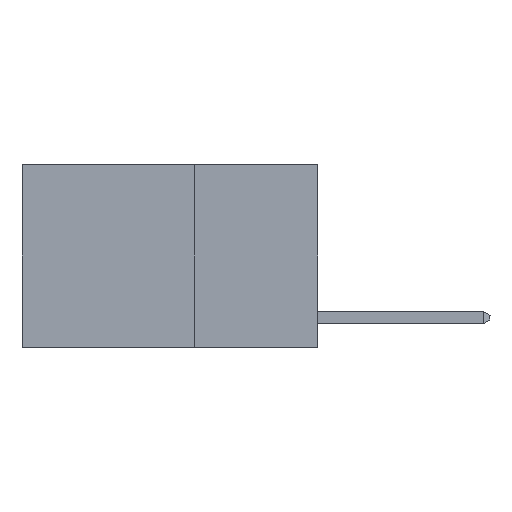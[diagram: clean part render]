
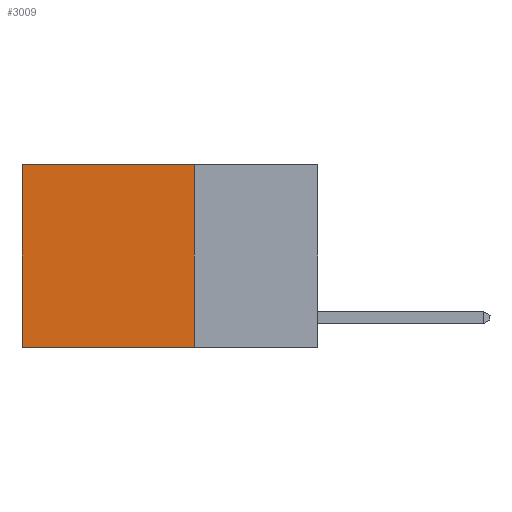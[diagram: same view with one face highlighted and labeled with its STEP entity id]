
A CAD part, left-side view. The second image highlights one B-rep face of the part: STEP entity #3009.
In plain terms, the highlighted planar face has unit normal (-1, 0, 0).
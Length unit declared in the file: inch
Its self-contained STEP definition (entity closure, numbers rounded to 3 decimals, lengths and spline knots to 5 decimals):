
#462 = LINE ( 'NONE', #7284, #9658 ) ;
#715 = VERTEX_POINT ( 'NONE', #5923 ) ;
#879 = AXIS2_PLACEMENT_3D ( 'NONE', #6379, #951, #7231 ) ;
#911 = EDGE_CURVE ( 'NONE', #4923, #715, #462, .T. ) ;
#945 = ORIENTED_EDGE ( 'NONE', *, *, #1492, .T. ) ;
#951 = DIRECTION ( 'NONE',  ( 1., 0., 0. ) ) ;
#1156 = LINE ( 'NONE', #4489, #3447 ) ;
#1469 = CARTESIAN_POINT ( 'NONE',  ( 0.2625, 0.6, 0. ) ) ;
#1492 = EDGE_CURVE ( 'NONE', #6433, #715, #4643, .T. ) ;
#1773 = EDGE_CURVE ( 'NONE', #6841, #4923, #7531, .T. ) ;
#1818 = VECTOR ( 'NONE', #6863, 39.37008 ) ;
#1923 = ORIENTED_EDGE ( 'NONE', *, *, #5623, .T. ) ;
#2501 = CARTESIAN_POINT ( 'NONE',  ( 0.2625, 0.25, 0. ) ) ;
#2544 = DIRECTION ( 'NONE',  ( 0., 0., -1. ) ) ;
#2850 = FACE_OUTER_BOUND ( 'NONE', #7343, .T. ) ;
#2915 = VECTOR ( 'NONE', #2544, 39.37008 ) ;
#3009 = ADVANCED_FACE ( 'NONE', ( #2850 ), #10342, .F. ) ;
#3053 = ORIENTED_EDGE ( 'NONE', *, *, #1773, .F. ) ;
#3447 = VECTOR ( 'NONE', #10206, 39.37008 ) ;
#4489 = CARTESIAN_POINT ( 'NONE',  ( 0.2625, 0.25, 0. ) ) ;
#4643 = LINE ( 'NONE', #7136, #1818 ) ;
#4923 = VERTEX_POINT ( 'NONE', #8606 ) ;
#5623 = EDGE_CURVE ( 'NONE', #6841, #6433, #1156, .T. ) ;
#5923 = CARTESIAN_POINT ( 'NONE',  ( 0.2625, 0.6, -0.37 ) ) ;
#6379 = CARTESIAN_POINT ( 'NONE',  ( 0.2625, 0.25, 0. ) ) ;
#6428 = DIRECTION ( 'NONE',  ( 0., 1., 0. ) ) ;
#6433 = VERTEX_POINT ( 'NONE', #1469 ) ;
#6841 = VERTEX_POINT ( 'NONE', #8933 ) ;
#6863 = DIRECTION ( 'NONE',  ( 0., 0., -1. ) ) ;
#7136 = CARTESIAN_POINT ( 'NONE',  ( 0.2625, 0.6, 0. ) ) ;
#7231 = DIRECTION ( 'NONE',  ( 0., 0., -1. ) ) ;
#7284 = CARTESIAN_POINT ( 'NONE',  ( 0.2625, 0.25, -0.37 ) ) ;
#7343 = EDGE_LOOP ( 'NONE', ( #945, #9735, #3053, #1923 ) ) ;
#7531 = LINE ( 'NONE', #2501, #2915 ) ;
#8606 = CARTESIAN_POINT ( 'NONE',  ( 0.2625, 0.25, -0.37 ) ) ;
#8933 = CARTESIAN_POINT ( 'NONE',  ( 0.2625, 0.25, 0. ) ) ;
#9658 = VECTOR ( 'NONE', #6428, 39.37008 ) ;
#9735 = ORIENTED_EDGE ( 'NONE', *, *, #911, .F. ) ;
#10206 = DIRECTION ( 'NONE',  ( 0., 1., 0. ) ) ;
#10342 = PLANE ( 'NONE',  #879 ) ;
